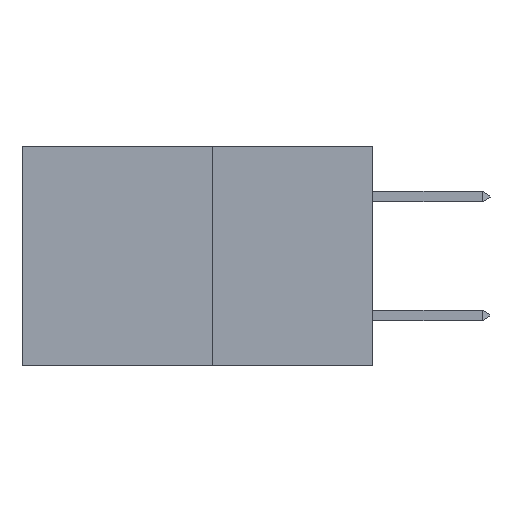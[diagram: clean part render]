
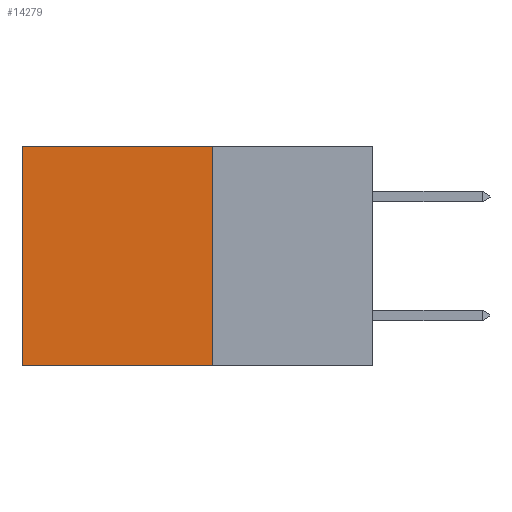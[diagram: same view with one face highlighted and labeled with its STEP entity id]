
A CAD part, left-side view. The second image highlights one B-rep face of the part: STEP entity #14279.
In plain terms, the highlighted planar face has unit normal (-1, 0, 0).
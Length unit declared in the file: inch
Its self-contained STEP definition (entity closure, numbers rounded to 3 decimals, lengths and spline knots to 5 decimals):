
#2939 = ORIENTED_EDGE ( 'NONE', *, *, #7929, .F. ) ;
#3095 = ORIENTED_EDGE ( 'NONE', *, *, #15422, .T. ) ;
#3167 = LINE ( 'NONE', #3558, #17025 ) ;
#3558 = CARTESIAN_POINT ( 'NONE',  ( 0.277, 0.59, -0.37 ) ) ;
#3602 = DIRECTION ( 'NONE',  ( 0., 1., 0. ) ) ;
#4357 = ORIENTED_EDGE ( 'NONE', *, *, #12690, .T. ) ;
#4388 = CARTESIAN_POINT ( 'NONE',  ( 0.277, 0.27, -0.37 ) ) ;
#5200 = ORIENTED_EDGE ( 'NONE', *, *, #17073, .F. ) ;
#5448 = PLANE ( 'NONE',  #11602 ) ;
#5503 = CARTESIAN_POINT ( 'NONE',  ( 0.277, 0.27, -0.37 ) ) ;
#5585 = CARTESIAN_POINT ( 'NONE',  ( 0.277, 0.59, -0.37 ) ) ;
#5736 = LINE ( 'NONE', #13287, #13538 ) ;
#5803 = DIRECTION ( 'NONE',  ( 0., 1., 0. ) ) ;
#5833 = VERTEX_POINT ( 'NONE', #14565 ) ;
#6009 = FACE_OUTER_BOUND ( 'NONE', #16764, .T. ) ;
#6891 = DIRECTION ( 'NONE',  ( 0., 0., -1. ) ) ;
#6934 = CARTESIAN_POINT ( 'NONE',  ( 0.277, 0.27, -0.37 ) ) ;
#7853 = VECTOR ( 'NONE', #5803, 39.37008 ) ;
#7929 = EDGE_CURVE ( 'NONE', #13483, #5833, #13494, .T. ) ;
#8570 = CARTESIAN_POINT ( 'NONE',  ( 0.277, 0.59, 0. ) ) ;
#10517 = DIRECTION ( 'NONE',  ( 0., 0., -1. ) ) ;
#10759 = VERTEX_POINT ( 'NONE', #8570 ) ;
#11534 = LINE ( 'NONE', #4388, #7853 ) ;
#11602 = AXIS2_PLACEMENT_3D ( 'NONE', #5503, #15205, #6891 ) ;
#12690 = EDGE_CURVE ( 'NONE', #10759, #16293, #3167, .T. ) ;
#13287 = CARTESIAN_POINT ( 'NONE',  ( 0.277, 0.27, 0. ) ) ;
#13483 = VERTEX_POINT ( 'NONE', #16474 ) ;
#13494 = LINE ( 'NONE', #6934, #17117 ) ;
#13538 = VECTOR ( 'NONE', #3602, 39.37008 ) ;
#14279 = ADVANCED_FACE ( 'NONE', ( #6009 ), #5448, .F. ) ;
#14565 = CARTESIAN_POINT ( 'NONE',  ( 0.277, 0.27, -0.37 ) ) ;
#15205 = DIRECTION ( 'NONE',  ( 1., 0., 0. ) ) ;
#15422 = EDGE_CURVE ( 'NONE', #13483, #10759, #5736, .T. ) ;
#16293 = VERTEX_POINT ( 'NONE', #5585 ) ;
#16474 = CARTESIAN_POINT ( 'NONE',  ( 0.277, 0.27, 0. ) ) ;
#16603 = DIRECTION ( 'NONE',  ( 0., 0., -1. ) ) ;
#16764 = EDGE_LOOP ( 'NONE', ( #4357, #5200, #2939, #3095 ) ) ;
#17025 = VECTOR ( 'NONE', #10517, 39.37008 ) ;
#17073 = EDGE_CURVE ( 'NONE', #5833, #16293, #11534, .T. ) ;
#17117 = VECTOR ( 'NONE', #16603, 39.37008 ) ;
